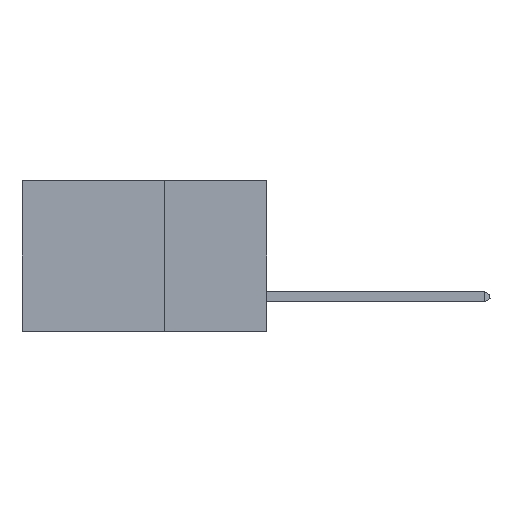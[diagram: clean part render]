
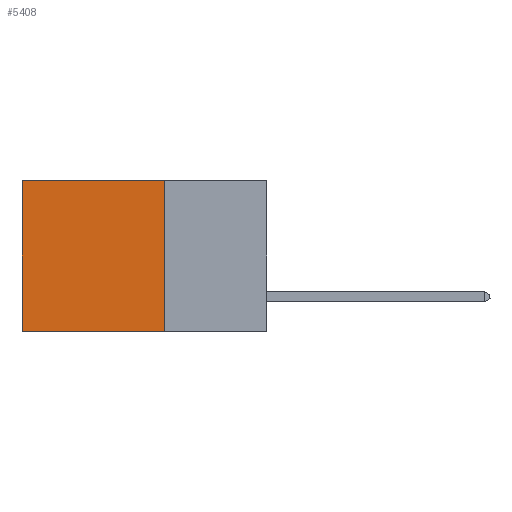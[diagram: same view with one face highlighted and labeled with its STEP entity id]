
A CAD part, left-side view. The second image highlights one B-rep face of the part: STEP entity #5408.
In plain terms, the highlighted planar face has unit normal (-1, 0, 0).
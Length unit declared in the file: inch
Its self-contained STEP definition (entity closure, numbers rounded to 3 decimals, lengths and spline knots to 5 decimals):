
#949 = FACE_OUTER_BOUND ( 'NONE', #4823, .T. ) ;
#2764 = VECTOR ( 'NONE', #13236, 39.37008 ) ;
#3159 = CARTESIAN_POINT ( 'NONE',  ( 0.2875, 0.6, -0.37 ) ) ;
#4020 = CARTESIAN_POINT ( 'NONE',  ( 0.2875, 0.25, -0.37 ) ) ;
#4823 = EDGE_LOOP ( 'NONE', ( #22647, #26096, #22392, #7027 ) ) ;
#5322 = CARTESIAN_POINT ( 'NONE',  ( 0.2875, 0.6, 0. ) ) ;
#5408 = ADVANCED_FACE ( 'NONE', ( #949 ), #24165, .F. ) ;
#6036 = VECTOR ( 'NONE', #15022, 39.37008 ) ;
#6209 = LINE ( 'NONE', #13433, #7497 ) ;
#6548 = CARTESIAN_POINT ( 'NONE',  ( 0.2875, 0.25, 0. ) ) ;
#7027 = ORIENTED_EDGE ( 'NONE', *, *, #17412, .T. ) ;
#7112 = VERTEX_POINT ( 'NONE', #10760 ) ;
#7206 = EDGE_CURVE ( 'NONE', #7112, #16623, #9614, .T. ) ;
#7423 = DIRECTION ( 'NONE',  ( 0., 0., -1. ) ) ;
#7497 = VECTOR ( 'NONE', #26317, 39.37008 ) ;
#9614 = LINE ( 'NONE', #5322, #20521 ) ;
#10760 = CARTESIAN_POINT ( 'NONE',  ( 0.2875, 0.6, 0. ) ) ;
#13236 = DIRECTION ( 'NONE',  ( 0., 0., -1. ) ) ;
#13433 = CARTESIAN_POINT ( 'NONE',  ( 0.2875, 0.25, -0.37 ) ) ;
#13529 = EDGE_CURVE ( 'NONE', #24425, #20644, #15656, .T. ) ;
#13988 = DIRECTION ( 'NONE',  ( 0., 0., -1. ) ) ;
#15022 = DIRECTION ( 'NONE',  ( 0., 1., 0. ) ) ;
#15625 = LINE ( 'NONE', #6548, #6036 ) ;
#15656 = LINE ( 'NONE', #17273, #2764 ) ;
#16623 = VERTEX_POINT ( 'NONE', #3159 ) ;
#17273 = CARTESIAN_POINT ( 'NONE',  ( 0.2875, 0.25, 0. ) ) ;
#17412 = EDGE_CURVE ( 'NONE', #24425, #7112, #15625, .T. ) ;
#20521 = VECTOR ( 'NONE', #7423, 39.37008 ) ;
#20644 = VERTEX_POINT ( 'NONE', #4020 ) ;
#21070 = CARTESIAN_POINT ( 'NONE',  ( 0.2875, 0.25, 0. ) ) ;
#21681 = AXIS2_PLACEMENT_3D ( 'NONE', #22044, #26232, #13988 ) ;
#22044 = CARTESIAN_POINT ( 'NONE',  ( 0.2875, 0.25, 0. ) ) ;
#22392 = ORIENTED_EDGE ( 'NONE', *, *, #13529, .F. ) ;
#22647 = ORIENTED_EDGE ( 'NONE', *, *, #7206, .T. ) ;
#24165 = PLANE ( 'NONE',  #21681 ) ;
#24425 = VERTEX_POINT ( 'NONE', #21070 ) ;
#26020 = EDGE_CURVE ( 'NONE', #20644, #16623, #6209, .T. ) ;
#26096 = ORIENTED_EDGE ( 'NONE', *, *, #26020, .F. ) ;
#26232 = DIRECTION ( 'NONE',  ( 1., 0., 0. ) ) ;
#26317 = DIRECTION ( 'NONE',  ( 0., 1., 0. ) ) ;
